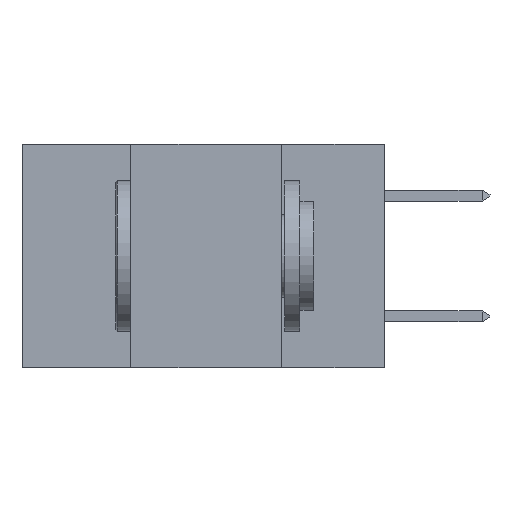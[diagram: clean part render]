
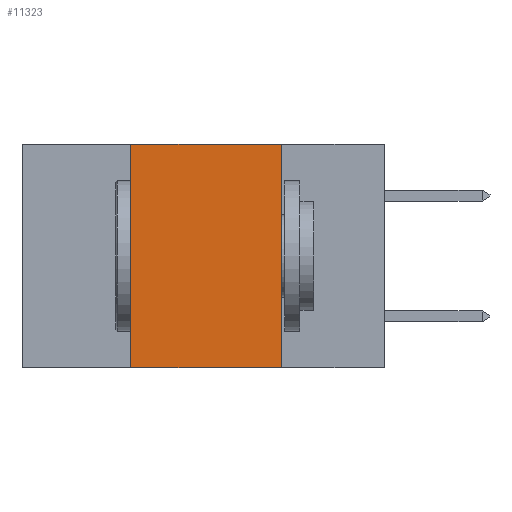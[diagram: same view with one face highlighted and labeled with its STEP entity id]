
A CAD part, left-side view. The second image highlights one B-rep face of the part: STEP entity #11323.
In plain terms, the highlighted planar face has unit normal (-1, 0, 0).
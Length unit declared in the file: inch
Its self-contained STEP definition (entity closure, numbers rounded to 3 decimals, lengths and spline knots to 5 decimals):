
#322 = CARTESIAN_POINT ( 'NONE',  ( 0., 0.6, 0. ) ) ;
#694 = CARTESIAN_POINT ( 'NONE',  ( 0., 0.17, 0. ) ) ;
#695 = VECTOR ( 'NONE', #4622, 39.37008 ) ;
#1313 = DIRECTION ( 'NONE',  ( 0., 0., -1. ) ) ;
#2449 = CARTESIAN_POINT ( 'NONE',  ( 0., 0.42, -0.37 ) ) ;
#2522 = CARTESIAN_POINT ( 'NONE',  ( 0., 0.6, 0. ) ) ;
#2589 = VECTOR ( 'NONE', #1313, 39.37008 ) ;
#2666 = CARTESIAN_POINT ( 'NONE',  ( 0., 0.42, 0. ) ) ;
#3273 = LINE ( 'NONE', #19379, #19144 ) ;
#4266 = ORIENTED_EDGE ( 'NONE', *, *, #5648, .T. ) ;
#4622 = DIRECTION ( 'NONE',  ( 0., -1., 0. ) ) ;
#4653 = LINE ( 'NONE', #2522, #17661 ) ;
#4821 = CARTESIAN_POINT ( 'NONE',  ( 0., 0.17, -0.37 ) ) ;
#4919 = EDGE_LOOP ( 'NONE', ( #12002, #8734, #19103, #4266 ) ) ;
#5648 = EDGE_CURVE ( 'NONE', #14095, #5675, #7355, .T. ) ;
#5675 = VERTEX_POINT ( 'NONE', #4821 ) ;
#5803 = DIRECTION ( 'NONE',  ( 0., 0., 1. ) ) ;
#6891 = EDGE_CURVE ( 'NONE', #7909, #18103, #4653, .T. ) ;
#6959 = DIRECTION ( 'NONE',  ( 0., -1., 0. ) ) ;
#7355 = LINE ( 'NONE', #16525, #695 ) ;
#7909 = VERTEX_POINT ( 'NONE', #2666 ) ;
#8734 = ORIENTED_EDGE ( 'NONE', *, *, #6891, .F. ) ;
#10035 = AXIS2_PLACEMENT_3D ( 'NONE', #322, #18368, #12442 ) ;
#10174 = CARTESIAN_POINT ( 'NONE',  ( 0., 0.17, 0. ) ) ;
#10420 = FACE_OUTER_BOUND ( 'NONE', #4919, .T. ) ;
#10640 = LINE ( 'NONE', #10174, #2589 ) ;
#11323 = ADVANCED_FACE ( 'NONE', ( #10420 ), #12316, .F. ) ;
#12002 = ORIENTED_EDGE ( 'NONE', *, *, #17681, .F. ) ;
#12316 = PLANE ( 'NONE',  #10035 ) ;
#12442 = DIRECTION ( 'NONE',  ( 0., 0., -1. ) ) ;
#14095 = VERTEX_POINT ( 'NONE', #2449 ) ;
#16525 = CARTESIAN_POINT ( 'NONE',  ( 0., 0.6, -0.37 ) ) ;
#17573 = EDGE_CURVE ( 'NONE', #14095, #7909, #3273, .T. ) ;
#17661 = VECTOR ( 'NONE', #6959, 39.37008 ) ;
#17681 = EDGE_CURVE ( 'NONE', #18103, #5675, #10640, .T. ) ;
#18103 = VERTEX_POINT ( 'NONE', #694 ) ;
#18368 = DIRECTION ( 'NONE',  ( 1., 0., 0. ) ) ;
#19103 = ORIENTED_EDGE ( 'NONE', *, *, #17573, .F. ) ;
#19144 = VECTOR ( 'NONE', #5803, 39.37008 ) ;
#19379 = CARTESIAN_POINT ( 'NONE',  ( 0., 0.42, 0. ) ) ;
